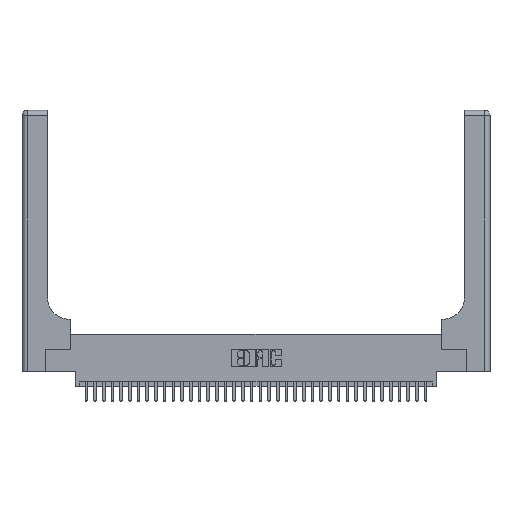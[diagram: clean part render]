
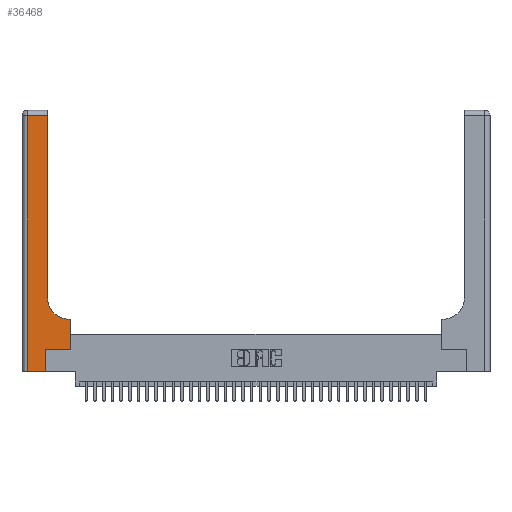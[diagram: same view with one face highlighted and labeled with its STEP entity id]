
A CAD part, top view. The second image highlights one B-rep face of the part: STEP entity #36468.
In plain terms, the highlighted planar face has unit normal (0, 0, 1).
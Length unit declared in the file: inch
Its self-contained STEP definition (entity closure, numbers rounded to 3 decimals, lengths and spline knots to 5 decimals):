
#401 = ORIENTED_EDGE ( 'NONE', *, *, #6642, .T. ) ;
#1332 = CARTESIAN_POINT ( 'NONE',  ( 0.06, 2.94, 0.37 ) ) ;
#1364 = VERTEX_POINT ( 'NONE', #23438 ) ;
#1394 = DIRECTION ( 'NONE',  ( 1., 0., 0. ) ) ;
#1691 = EDGE_CURVE ( 'NONE', #36826, #5670, #9582, .T. ) ;
#1743 = DIRECTION ( 'NONE',  ( 1., 0., 0. ) ) ;
#1836 = EDGE_CURVE ( 'NONE', #15995, #17411, #31594, .T. ) ;
#1973 = LINE ( 'NONE', #32578, #26139 ) ;
#2179 = ORIENTED_EDGE ( 'NONE', *, *, #35562, .T. ) ;
#3901 = ORIENTED_EDGE ( 'NONE', *, *, #1836, .T. ) ;
#3978 = AXIS2_PLACEMENT_3D ( 'NONE', #4350, #24493, #1394 ) ;
#4350 = CARTESIAN_POINT ( 'NONE',  ( 0.5415, 0.85, 0.37 ) ) ;
#4406 = CARTESIAN_POINT ( 'NONE',  ( 0.2915, 2.94, 0.37 ) ) ;
#5312 = CARTESIAN_POINT ( 'NONE',  ( 0.2915, 0.85, 0.37 ) ) ;
#5670 = VERTEX_POINT ( 'NONE', #10401 ) ;
#5774 = CARTESIAN_POINT ( 'NONE',  ( 0., 2.94, 0.37 ) ) ;
#5810 = CARTESIAN_POINT ( 'NONE',  ( 0.06, 0., 0.37 ) ) ;
#5848 = ORIENTED_EDGE ( 'NONE', *, *, #35329, .T. ) ;
#6642 = EDGE_CURVE ( 'NONE', #22027, #15995, #10848, .T. ) ;
#6880 = ORIENTED_EDGE ( 'NONE', *, *, #15112, .T. ) ;
#7032 = VECTOR ( 'NONE', #21395, 39.37008 ) ;
#8267 = DIRECTION ( 'NONE',  ( 0., 1., 0. ) ) ;
#8495 = VERTEX_POINT ( 'NONE', #1332 ) ;
#8638 = CARTESIAN_POINT ( 'NONE',  ( 0.269, 0., 0.37 ) ) ;
#8745 = VECTOR ( 'NONE', #1743, 39.37008 ) ;
#9294 = LINE ( 'NONE', #21035, #23171 ) ;
#9347 = VECTOR ( 'NONE', #30681, 39.37008 ) ;
#9582 = LINE ( 'NONE', #33062, #8745 ) ;
#10245 = VECTOR ( 'NONE', #19805, 39.37008 ) ;
#10401 = CARTESIAN_POINT ( 'NONE',  ( 0.5585, 0.25, 0.37 ) ) ;
#10848 = CIRCLE ( 'NONE', #3978, 0.25 ) ;
#11842 = CARTESIAN_POINT ( 'NONE',  ( 0., 3., 0.37 ) ) ;
#11949 = DIRECTION ( 'NONE',  ( 0., 0., -1. ) ) ;
#12944 = DIRECTION ( 'NONE',  ( 0., 1., 0. ) ) ;
#14804 = PLANE ( 'NONE',  #27577 ) ;
#15030 = FACE_OUTER_BOUND ( 'NONE', #17595, .T. ) ;
#15112 = EDGE_CURVE ( 'NONE', #36303, #36826, #1973, .T. ) ;
#15995 = VERTEX_POINT ( 'NONE', #5312 ) ;
#17383 = EDGE_CURVE ( 'NONE', #8495, #23907, #20463, .T. ) ;
#17411 = VERTEX_POINT ( 'NONE', #4406 ) ;
#17595 = EDGE_LOOP ( 'NONE', ( #3901, #2179, #20609, #28603, #6880, #34355, #26201, #5848, #401 ) ) ;
#19550 = CARTESIAN_POINT ( 'NONE',  ( 0.2915, 0.6, 0.37 ) ) ;
#19805 = DIRECTION ( 'NONE',  ( -1., 0., 0. ) ) ;
#19942 = VECTOR ( 'NONE', #12944, 39.37008 ) ;
#20463 = LINE ( 'NONE', #27434, #7032 ) ;
#20559 = DIRECTION ( 'NONE',  ( 1., 0., 0. ) ) ;
#20609 = ORIENTED_EDGE ( 'NONE', *, *, #17383, .T. ) ;
#21035 = CARTESIAN_POINT ( 'NONE',  ( 0.5585, 0.25, 0.37 ) ) ;
#21395 = DIRECTION ( 'NONE',  ( 0., -1., 0. ) ) ;
#22027 = VERTEX_POINT ( 'NONE', #37001 ) ;
#23171 = VECTOR ( 'NONE', #29927, 39.37008 ) ;
#23438 = CARTESIAN_POINT ( 'NONE',  ( 0.5585, 0.6, 0.37 ) ) ;
#23907 = VERTEX_POINT ( 'NONE', #5810 ) ;
#24493 = DIRECTION ( 'NONE',  ( 0., 0., -1. ) ) ;
#26139 = VECTOR ( 'NONE', #8267, 39.37008 ) ;
#26201 = ORIENTED_EDGE ( 'NONE', *, *, #26656, .T. ) ;
#26656 = EDGE_CURVE ( 'NONE', #5670, #1364, #9294, .T. ) ;
#27221 = CARTESIAN_POINT ( 'NONE',  ( 0.2915, 3., 0.37 ) ) ;
#27434 = CARTESIAN_POINT ( 'NONE',  ( 0.06, 3., 0.37 ) ) ;
#27577 = AXIS2_PLACEMENT_3D ( 'NONE', #11842, #11949, #35220 ) ;
#27706 = LINE ( 'NONE', #34629, #31317 ) ;
#28603 = ORIENTED_EDGE ( 'NONE', *, *, #29714, .T. ) ;
#29714 = EDGE_CURVE ( 'NONE', #23907, #36303, #27706, .T. ) ;
#29927 = DIRECTION ( 'NONE',  ( 0., 1., 0. ) ) ;
#30681 = DIRECTION ( 'NONE',  ( -1., 0., 0. ) ) ;
#31317 = VECTOR ( 'NONE', #20559, 39.37008 ) ;
#31594 = LINE ( 'NONE', #27221, #19942 ) ;
#32578 = CARTESIAN_POINT ( 'NONE',  ( 0.269, 0., 0.37 ) ) ;
#33062 = CARTESIAN_POINT ( 'NONE',  ( 0.269, 0.25, 0.37 ) ) ;
#33090 = CARTESIAN_POINT ( 'NONE',  ( 0.269, 0.25, 0.37 ) ) ;
#33568 = LINE ( 'NONE', #5774, #10245 ) ;
#34044 = LINE ( 'NONE', #19550, #9347 ) ;
#34355 = ORIENTED_EDGE ( 'NONE', *, *, #1691, .T. ) ;
#34629 = CARTESIAN_POINT ( 'NONE',  ( 0., 0., 0.37 ) ) ;
#35220 = DIRECTION ( 'NONE',  ( -1., 0., 0. ) ) ;
#35329 = EDGE_CURVE ( 'NONE', #1364, #22027, #34044, .T. ) ;
#35562 = EDGE_CURVE ( 'NONE', #17411, #8495, #33568, .T. ) ;
#36303 = VERTEX_POINT ( 'NONE', #8638 ) ;
#36468 = ADVANCED_FACE ( 'NONE', ( #15030 ), #14804, .F. ) ;
#36826 = VERTEX_POINT ( 'NONE', #33090 ) ;
#37001 = CARTESIAN_POINT ( 'NONE',  ( 0.5415, 0.6, 0.37 ) ) ;
